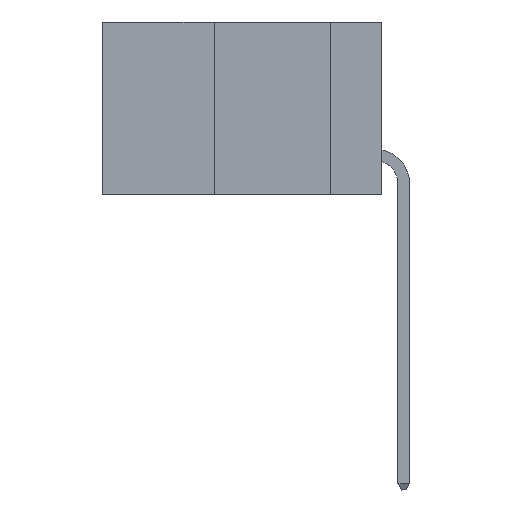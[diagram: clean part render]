
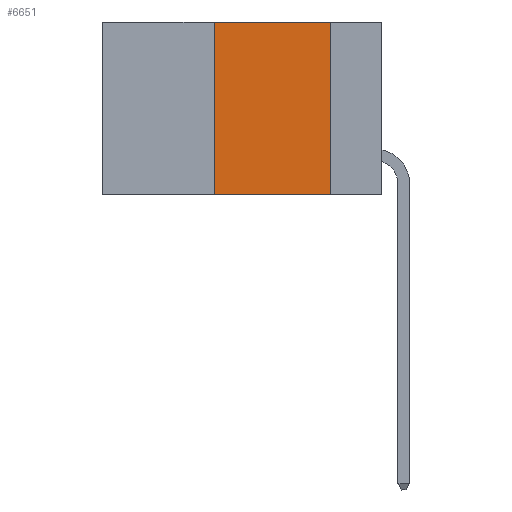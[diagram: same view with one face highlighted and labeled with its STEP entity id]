
A CAD part, left-side view. The second image highlights one B-rep face of the part: STEP entity #6651.
In plain terms, the highlighted planar face has unit normal (-1, 0, 0).
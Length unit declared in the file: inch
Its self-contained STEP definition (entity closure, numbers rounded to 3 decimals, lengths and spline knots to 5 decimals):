
#278 = EDGE_CURVE ( 'NONE', #13788, #11509, #17261, .T. ) ;
#481 = VECTOR ( 'NONE', #9909, 39.37008 ) ;
#1640 = DIRECTION ( 'NONE',  ( 0., 0., 1. ) ) ;
#2387 = VECTOR ( 'NONE', #8651, 39.37008 ) ;
#3653 = CARTESIAN_POINT ( 'NONE',  ( 0., 0.11, 0. ) ) ;
#3921 = LINE ( 'NONE', #9110, #19186 ) ;
#5602 = VERTEX_POINT ( 'NONE', #16831 ) ;
#6651 = ADVANCED_FACE ( 'NONE', ( #19016 ), #11297, .F. ) ;
#7152 = CARTESIAN_POINT ( 'NONE',  ( 0., 0.6, -0.37 ) ) ;
#8077 = EDGE_LOOP ( 'NONE', ( #10845, #11228, #11921, #15308 ) ) ;
#8651 = DIRECTION ( 'NONE',  ( 0., -1., 0. ) ) ;
#9110 = CARTESIAN_POINT ( 'NONE',  ( 0., 0.6, 0. ) ) ;
#9300 = VERTEX_POINT ( 'NONE', #3653 ) ;
#9413 = VECTOR ( 'NONE', #1640, 39.37008 ) ;
#9909 = DIRECTION ( 'NONE',  ( 0., 0., -1. ) ) ;
#10845 = ORIENTED_EDGE ( 'NONE', *, *, #11732, .F. ) ;
#11050 = DIRECTION ( 'NONE',  ( 0., 0., -1. ) ) ;
#11078 = DIRECTION ( 'NONE',  ( 1., 0., 0. ) ) ;
#11203 = CARTESIAN_POINT ( 'NONE',  ( 0., 0.6, 0. ) ) ;
#11228 = ORIENTED_EDGE ( 'NONE', *, *, #18789, .F. ) ;
#11297 = PLANE ( 'NONE',  #16546 ) ;
#11432 = CARTESIAN_POINT ( 'NONE',  ( 0., 0.11, 0. ) ) ;
#11509 = VERTEX_POINT ( 'NONE', #15329 ) ;
#11732 = EDGE_CURVE ( 'NONE', #9300, #5602, #12844, .T. ) ;
#11921 = ORIENTED_EDGE ( 'NONE', *, *, #278, .F. ) ;
#12844 = LINE ( 'NONE', #11432, #481 ) ;
#13788 = VERTEX_POINT ( 'NONE', #17299 ) ;
#14605 = LINE ( 'NONE', #7152, #2387 ) ;
#15096 = EDGE_CURVE ( 'NONE', #13788, #5602, #14605, .T. ) ;
#15308 = ORIENTED_EDGE ( 'NONE', *, *, #15096, .T. ) ;
#15329 = CARTESIAN_POINT ( 'NONE',  ( 0., 0.36, 0. ) ) ;
#15837 = CARTESIAN_POINT ( 'NONE',  ( 0., 0.36, 0. ) ) ;
#16546 = AXIS2_PLACEMENT_3D ( 'NONE', #11203, #11078, #11050 ) ;
#16579 = DIRECTION ( 'NONE',  ( 0., -1., 0. ) ) ;
#16831 = CARTESIAN_POINT ( 'NONE',  ( 0., 0.11, -0.37 ) ) ;
#17261 = LINE ( 'NONE', #15837, #9413 ) ;
#17299 = CARTESIAN_POINT ( 'NONE',  ( 0., 0.36, -0.37 ) ) ;
#18789 = EDGE_CURVE ( 'NONE', #11509, #9300, #3921, .T. ) ;
#19016 = FACE_OUTER_BOUND ( 'NONE', #8077, .T. ) ;
#19186 = VECTOR ( 'NONE', #16579, 39.37008 ) ;
